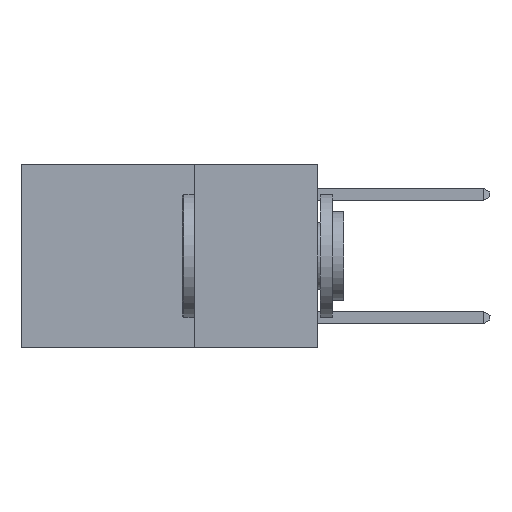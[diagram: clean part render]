
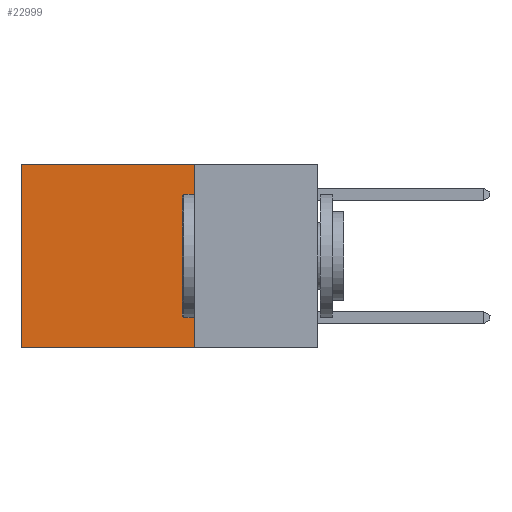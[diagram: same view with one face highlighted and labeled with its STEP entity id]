
A CAD part, left-side view. The second image highlights one B-rep face of the part: STEP entity #22999.
In plain terms, the highlighted planar face has unit normal (-1, 0, 0).
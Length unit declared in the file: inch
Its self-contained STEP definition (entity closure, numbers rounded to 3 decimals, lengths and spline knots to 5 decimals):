
#205 = DIRECTION ( 'NONE',  ( 0., 0., -1. ) ) ;
#239 = CARTESIAN_POINT ( 'NONE',  ( 0.2625, 0.25, -0.37 ) ) ;
#325 = CARTESIAN_POINT ( 'NONE',  ( 0.2625, 0.6, 0. ) ) ;
#2040 = EDGE_CURVE ( 'NONE', #21329, #8507, #8737, .T. ) ;
#3006 = VECTOR ( 'NONE', #9633, 39.37008 ) ;
#4015 = EDGE_CURVE ( 'NONE', #8507, #21048, #13311, .T. ) ;
#5806 = EDGE_CURVE ( 'NONE', #26243, #21048, #9210, .T. ) ;
#6161 = LINE ( 'NONE', #22326, #17836 ) ;
#6884 = CARTESIAN_POINT ( 'NONE',  ( 0.2625, 0.25, 0. ) ) ;
#7272 = VECTOR ( 'NONE', #15645, 39.37008 ) ;
#7456 = ORIENTED_EDGE ( 'NONE', *, *, #5806, .T. ) ;
#7867 = VECTOR ( 'NONE', #10944, 39.37008 ) ;
#8376 = AXIS2_PLACEMENT_3D ( 'NONE', #16316, #14172, #205 ) ;
#8507 = VERTEX_POINT ( 'NONE', #239 ) ;
#8737 = LINE ( 'NONE', #29207, #7272 ) ;
#9210 = LINE ( 'NONE', #325, #3006 ) ;
#9633 = DIRECTION ( 'NONE',  ( 0., 0., -1. ) ) ;
#10559 = CARTESIAN_POINT ( 'NONE',  ( 0.2625, 0.6, -0.37 ) ) ;
#10944 = DIRECTION ( 'NONE',  ( 0., 1., 0. ) ) ;
#11100 = CARTESIAN_POINT ( 'NONE',  ( 0.2625, 0.6, 0. ) ) ;
#13271 = CARTESIAN_POINT ( 'NONE',  ( 0.2625, 0.25, -0.37 ) ) ;
#13311 = LINE ( 'NONE', #13271, #7867 ) ;
#14172 = DIRECTION ( 'NONE',  ( 1., 0., 0. ) ) ;
#15645 = DIRECTION ( 'NONE',  ( 0., 0., -1. ) ) ;
#16316 = CARTESIAN_POINT ( 'NONE',  ( 0.2625, 0.25, 0. ) ) ;
#17710 = ORIENTED_EDGE ( 'NONE', *, *, #27383, .T. ) ;
#17836 = VECTOR ( 'NONE', #24571, 39.37008 ) ;
#17980 = ORIENTED_EDGE ( 'NONE', *, *, #2040, .F. ) ;
#20160 = EDGE_LOOP ( 'NONE', ( #7456, #22128, #17980, #17710 ) ) ;
#21048 = VERTEX_POINT ( 'NONE', #10559 ) ;
#21329 = VERTEX_POINT ( 'NONE', #6884 ) ;
#22128 = ORIENTED_EDGE ( 'NONE', *, *, #4015, .F. ) ;
#22326 = CARTESIAN_POINT ( 'NONE',  ( 0.2625, 0.25, 0. ) ) ;
#22999 = ADVANCED_FACE ( 'NONE', ( #24976 ), #23288, .F. ) ;
#23288 = PLANE ( 'NONE',  #8376 ) ;
#24571 = DIRECTION ( 'NONE',  ( 0., 1., 0. ) ) ;
#24976 = FACE_OUTER_BOUND ( 'NONE', #20160, .T. ) ;
#26243 = VERTEX_POINT ( 'NONE', #11100 ) ;
#27383 = EDGE_CURVE ( 'NONE', #21329, #26243, #6161, .T. ) ;
#29207 = CARTESIAN_POINT ( 'NONE',  ( 0.2625, 0.25, 0. ) ) ;
